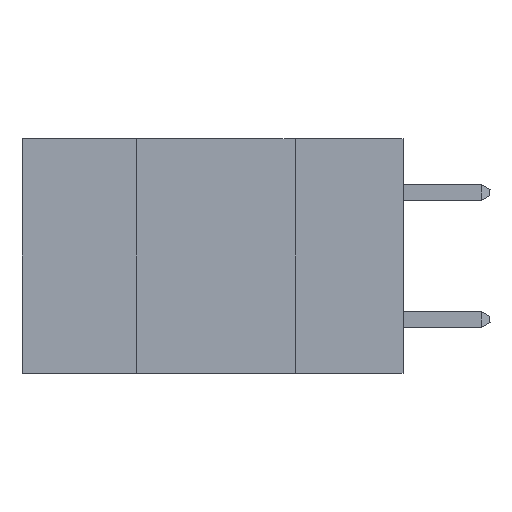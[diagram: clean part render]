
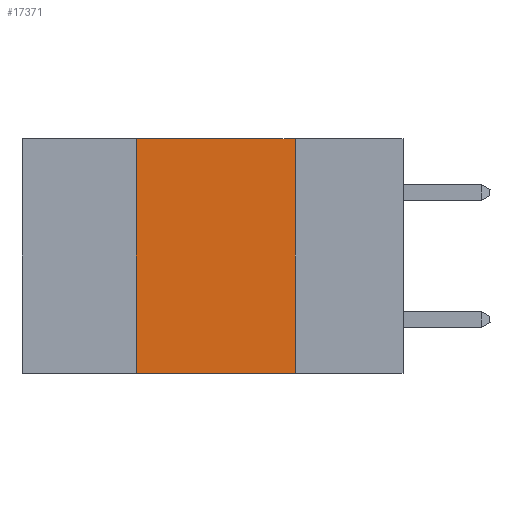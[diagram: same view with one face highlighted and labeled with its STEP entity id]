
A CAD part, left-side view. The second image highlights one B-rep face of the part: STEP entity #17371.
In plain terms, the highlighted planar face has unit normal (-1, 0, 0).
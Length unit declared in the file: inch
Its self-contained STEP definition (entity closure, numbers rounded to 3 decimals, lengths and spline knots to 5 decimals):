
#464 = DIRECTION ( 'NONE',  ( 0., 0., -1. ) ) ;
#1051 = AXIS2_PLACEMENT_3D ( 'NONE', #16332, #22398, #10242 ) ;
#2311 = ORIENTED_EDGE ( 'NONE', *, *, #17594, .F. ) ;
#2371 = ORIENTED_EDGE ( 'NONE', *, *, #21135, .F. ) ;
#2706 = ORIENTED_EDGE ( 'NONE', *, *, #13649, .F. ) ;
#2806 = CARTESIAN_POINT ( 'NONE',  ( 0., 0.42, 0. ) ) ;
#2913 = ORIENTED_EDGE ( 'NONE', *, *, #12985, .T. ) ;
#3259 = LINE ( 'NONE', #8457, #19077 ) ;
#3643 = DIRECTION ( 'NONE',  ( 0., -1., 0. ) ) ;
#4878 = VERTEX_POINT ( 'NONE', #13835 ) ;
#4945 = VECTOR ( 'NONE', #3643, 39.37008 ) ;
#8457 = CARTESIAN_POINT ( 'NONE',  ( 0., 0.42, 0. ) ) ;
#9469 = VECTOR ( 'NONE', #22217, 39.37008 ) ;
#9859 = VERTEX_POINT ( 'NONE', #16547 ) ;
#10242 = DIRECTION ( 'NONE',  ( 0., 0., -1. ) ) ;
#10468 = LINE ( 'NONE', #14075, #4945 ) ;
#10929 = VERTEX_POINT ( 'NONE', #11471 ) ;
#11471 = CARTESIAN_POINT ( 'NONE',  ( 0., 0.42, -0.37 ) ) ;
#12059 = EDGE_LOOP ( 'NONE', ( #2311, #2371, #2706, #2913 ) ) ;
#12985 = EDGE_CURVE ( 'NONE', #10929, #9859, #20946, .T. ) ;
#13649 = EDGE_CURVE ( 'NONE', #10929, #20870, #3259, .T. ) ;
#13835 = CARTESIAN_POINT ( 'NONE',  ( 0., 0.17, 0. ) ) ;
#14075 = CARTESIAN_POINT ( 'NONE',  ( 0., 0.6, 0. ) ) ;
#16129 = VECTOR ( 'NONE', #464, 39.37008 ) ;
#16332 = CARTESIAN_POINT ( 'NONE',  ( 0., 0.6, 0. ) ) ;
#16547 = CARTESIAN_POINT ( 'NONE',  ( 0., 0.17, -0.37 ) ) ;
#16635 = DIRECTION ( 'NONE',  ( 0., 0., 1. ) ) ;
#17009 = CARTESIAN_POINT ( 'NONE',  ( 0., 0.17, 0. ) ) ;
#17371 = ADVANCED_FACE ( 'NONE', ( #21814 ), #20403, .F. ) ;
#17594 = EDGE_CURVE ( 'NONE', #4878, #9859, #21492, .T. ) ;
#18215 = CARTESIAN_POINT ( 'NONE',  ( 0., 0.6, -0.37 ) ) ;
#19077 = VECTOR ( 'NONE', #16635, 39.37008 ) ;
#20403 = PLANE ( 'NONE',  #1051 ) ;
#20870 = VERTEX_POINT ( 'NONE', #2806 ) ;
#20946 = LINE ( 'NONE', #18215, #9469 ) ;
#21135 = EDGE_CURVE ( 'NONE', #20870, #4878, #10468, .T. ) ;
#21492 = LINE ( 'NONE', #17009, #16129 ) ;
#21814 = FACE_OUTER_BOUND ( 'NONE', #12059, .T. ) ;
#22217 = DIRECTION ( 'NONE',  ( 0., -1., 0. ) ) ;
#22398 = DIRECTION ( 'NONE',  ( 1., 0., 0. ) ) ;
